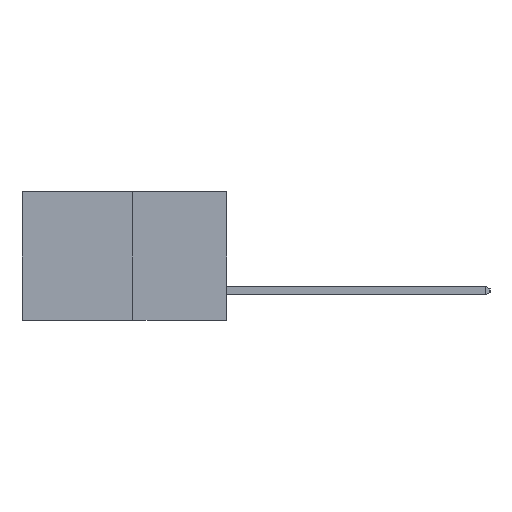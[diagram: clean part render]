
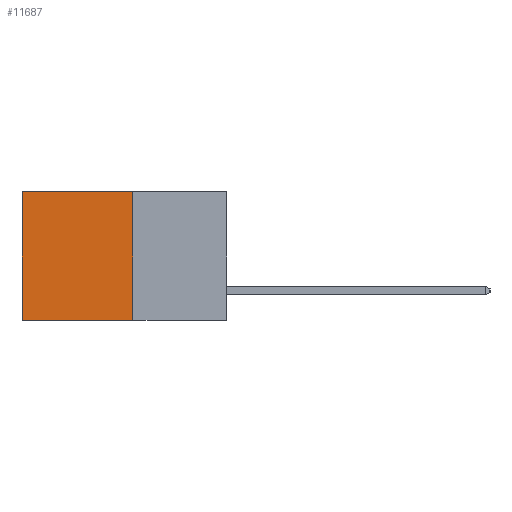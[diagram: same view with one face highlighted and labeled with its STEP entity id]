
A CAD part, left-side view. The second image highlights one B-rep face of the part: STEP entity #11687.
In plain terms, the highlighted planar face has unit normal (-1, 0, 0).
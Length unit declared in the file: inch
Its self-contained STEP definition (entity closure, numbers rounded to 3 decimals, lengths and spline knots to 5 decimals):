
#793 = EDGE_CURVE ( 'NONE', #15663, #7310, #7302, .T. ) ;
#914 = VERTEX_POINT ( 'NONE', #5866 ) ;
#1730 = VECTOR ( 'NONE', #13090, 39.37008 ) ;
#2606 = FACE_OUTER_BOUND ( 'NONE', #16580, .T. ) ;
#2862 = PLANE ( 'NONE',  #4600 ) ;
#3376 = CARTESIAN_POINT ( 'NONE',  ( 0.277, 0.59, -0.37 ) ) ;
#4600 = AXIS2_PLACEMENT_3D ( 'NONE', #11221, #7179, #16170 ) ;
#5607 = LINE ( 'NONE', #12845, #1730 ) ;
#5866 = CARTESIAN_POINT ( 'NONE',  ( 0.277, 0.59, 0. ) ) ;
#6388 = EDGE_CURVE ( 'NONE', #16090, #15663, #7464, .T. ) ;
#6868 = VECTOR ( 'NONE', #14840, 39.37008 ) ;
#7056 = CARTESIAN_POINT ( 'NONE',  ( 0.277, 0.27, -0.37 ) ) ;
#7179 = DIRECTION ( 'NONE',  ( 1., 0., 0. ) ) ;
#7302 = LINE ( 'NONE', #7056, #6868 ) ;
#7310 = VERTEX_POINT ( 'NONE', #3376 ) ;
#7464 = LINE ( 'NONE', #17191, #13986 ) ;
#8517 = DIRECTION ( 'NONE',  ( 0., 1., 0. ) ) ;
#8620 = CARTESIAN_POINT ( 'NONE',  ( 0.277, 0.27, 0. ) ) ;
#9459 = EDGE_CURVE ( 'NONE', #914, #7310, #5607, .T. ) ;
#9907 = EDGE_CURVE ( 'NONE', #16090, #914, #14437, .T. ) ;
#10018 = ORIENTED_EDGE ( 'NONE', *, *, #6388, .F. ) ;
#11002 = ORIENTED_EDGE ( 'NONE', *, *, #9907, .T. ) ;
#11170 = VECTOR ( 'NONE', #8517, 39.37008 ) ;
#11221 = CARTESIAN_POINT ( 'NONE',  ( 0.277, 0.27, -0.37 ) ) ;
#11228 = CARTESIAN_POINT ( 'NONE',  ( 0.277, 0.27, -0.37 ) ) ;
#11687 = ADVANCED_FACE ( 'NONE', ( #2606 ), #2862, .F. ) ;
#12845 = CARTESIAN_POINT ( 'NONE',  ( 0.277, 0.59, -0.37 ) ) ;
#13090 = DIRECTION ( 'NONE',  ( 0., 0., -1. ) ) ;
#13200 = CARTESIAN_POINT ( 'NONE',  ( 0.277, 0.27, 0. ) ) ;
#13986 = VECTOR ( 'NONE', #17140, 39.37008 ) ;
#14437 = LINE ( 'NONE', #8620, #11170 ) ;
#14840 = DIRECTION ( 'NONE',  ( 0., 1., 0. ) ) ;
#14956 = ORIENTED_EDGE ( 'NONE', *, *, #9459, .T. ) ;
#15663 = VERTEX_POINT ( 'NONE', #11228 ) ;
#16090 = VERTEX_POINT ( 'NONE', #13200 ) ;
#16170 = DIRECTION ( 'NONE',  ( 0., 0., -1. ) ) ;
#16576 = ORIENTED_EDGE ( 'NONE', *, *, #793, .F. ) ;
#16580 = EDGE_LOOP ( 'NONE', ( #14956, #16576, #10018, #11002 ) ) ;
#17140 = DIRECTION ( 'NONE',  ( 0., 0., -1. ) ) ;
#17191 = CARTESIAN_POINT ( 'NONE',  ( 0.277, 0.27, -0.37 ) ) ;
